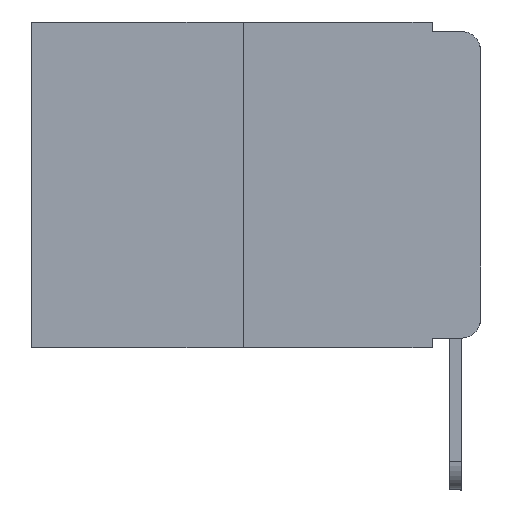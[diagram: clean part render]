
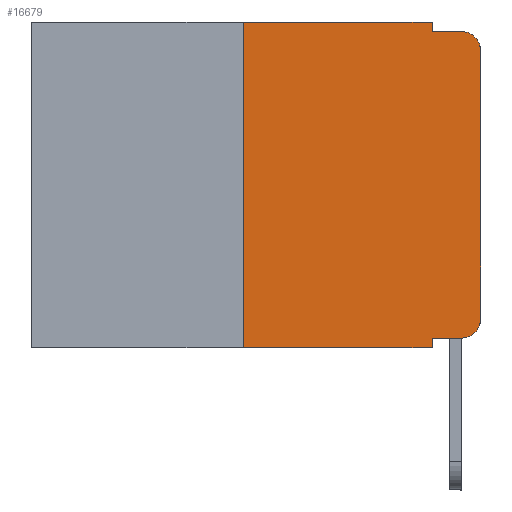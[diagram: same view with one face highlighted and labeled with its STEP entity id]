
A CAD part, left-side view. The second image highlights one B-rep face of the part: STEP entity #16679.
In plain terms, the highlighted planar face has unit normal (-1, 0, 0).
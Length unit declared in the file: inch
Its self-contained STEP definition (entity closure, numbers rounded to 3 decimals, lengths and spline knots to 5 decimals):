
#248 = LINE ( 'NONE', #6428, #6552 ) ;
#523 = EDGE_CURVE ( 'NONE', #12694, #17969, #16596, .T. ) ;
#1305 = VECTOR ( 'NONE', #3465, 39.37008 ) ;
#1343 = DIRECTION ( 'NONE',  ( 0., 0., -1. ) ) ;
#1413 = CARTESIAN_POINT ( 'NONE',  ( 0., 0., -0.03 ) ) ;
#1513 = CARTESIAN_POINT ( 'NONE',  ( 0., 0.473, -0.343 ) ) ;
#1950 = AXIS2_PLACEMENT_3D ( 'NONE', #7630, #7432, #1343 ) ;
#3198 = CARTESIAN_POINT ( 'NONE',  ( 0., 0.02, -0.333 ) ) ;
#3221 = EDGE_CURVE ( 'NONE', #6096, #13166, #12821, .T. ) ;
#3465 = DIRECTION ( 'NONE',  ( 0., 0., -1. ) ) ;
#3627 = ORIENTED_EDGE ( 'NONE', *, *, #523, .F. ) ;
#3660 = CARTESIAN_POINT ( 'NONE',  ( 0., 0.051, 0. ) ) ;
#3879 = CARTESIAN_POINT ( 'NONE',  ( 0., 0.25, -0.343 ) ) ;
#3908 = ORIENTED_EDGE ( 'NONE', *, *, #4370, .F. ) ;
#3960 = CIRCLE ( 'NONE', #19235, 0.02 ) ;
#4212 = CARTESIAN_POINT ( 'NONE',  ( 0., 0.25, 0. ) ) ;
#4370 = EDGE_CURVE ( 'NONE', #14528, #16670, #248, .T. ) ;
#4407 = VECTOR ( 'NONE', #10642, 39.37008 ) ;
#4657 = DIRECTION ( 'NONE',  ( 0., 0., 1. ) ) ;
#4726 = ORIENTED_EDGE ( 'NONE', *, *, #6955, .T. ) ;
#4811 = DIRECTION ( 'NONE',  ( -1., 0., 0. ) ) ;
#5202 = EDGE_CURVE ( 'NONE', #8210, #15841, #7798, .T. ) ;
#5448 = ORIENTED_EDGE ( 'NONE', *, *, #18384, .T. ) ;
#6096 = VERTEX_POINT ( 'NONE', #17494 ) ;
#6428 = CARTESIAN_POINT ( 'NONE',  ( 0., 0.051, 0. ) ) ;
#6497 = CARTESIAN_POINT ( 'NONE',  ( 0., 0.473, 0. ) ) ;
#6552 = VECTOR ( 'NONE', #17311, 39.37008 ) ;
#6747 = EDGE_LOOP ( 'NONE', ( #20002, #5448, #15507, #15849, #15012, #3627, #12566, #3908, #11914, #4726 ) ) ;
#6955 = EDGE_CURVE ( 'NONE', #18101, #8210, #16086, .T. ) ;
#7432 = DIRECTION ( 'NONE',  ( 1., 0., 0. ) ) ;
#7459 = CARTESIAN_POINT ( 'NONE',  ( 0., 0., -0.313 ) ) ;
#7630 = CARTESIAN_POINT ( 'NONE',  ( 0., 0.473, 0. ) ) ;
#7725 = DIRECTION ( 'NONE',  ( 0., -1., 0. ) ) ;
#7746 = CARTESIAN_POINT ( 'NONE',  ( 0., 0.02, -0.313 ) ) ;
#7798 = LINE ( 'NONE', #12476, #10838 ) ;
#8210 = VERTEX_POINT ( 'NONE', #7459 ) ;
#10475 = CARTESIAN_POINT ( 'NONE',  ( 0., 0.051, -0.343 ) ) ;
#10642 = DIRECTION ( 'NONE',  ( 0., -1., 0. ) ) ;
#10838 = VECTOR ( 'NONE', #4657, 39.37008 ) ;
#11497 = CARTESIAN_POINT ( 'NONE',  ( 0., 0.051, -0.01 ) ) ;
#11809 = CARTESIAN_POINT ( 'NONE',  ( 0., 0.25, 0. ) ) ;
#11914 = ORIENTED_EDGE ( 'NONE', *, *, #13280, .T. ) ;
#11916 = DIRECTION ( 'NONE',  ( 0., 0., 1. ) ) ;
#12083 = CARTESIAN_POINT ( 'NONE',  ( 0., 0.02, -0.03 ) ) ;
#12347 = VERTEX_POINT ( 'NONE', #13642 ) ;
#12476 = CARTESIAN_POINT ( 'NONE',  ( 0., 0., 0. ) ) ;
#12566 = ORIENTED_EDGE ( 'NONE', *, *, #13391, .T. ) ;
#12694 = VERTEX_POINT ( 'NONE', #3879 ) ;
#12783 = CARTESIAN_POINT ( 'NONE',  ( 0., 0.02, -0.01 ) ) ;
#12821 = LINE ( 'NONE', #11497, #15847 ) ;
#13166 = VERTEX_POINT ( 'NONE', #12783 ) ;
#13225 = DIRECTION ( 'NONE',  ( 0., -1., 0. ) ) ;
#13280 = EDGE_CURVE ( 'NONE', #14528, #18101, #18278, .T. ) ;
#13391 = EDGE_CURVE ( 'NONE', #12694, #16670, #16845, .T. ) ;
#13642 = CARTESIAN_POINT ( 'NONE',  ( 0., 0.051, 0. ) ) ;
#13929 = FACE_OUTER_BOUND ( 'NONE', #6747, .T. ) ;
#14127 = VECTOR ( 'NONE', #20014, 39.37008 ) ;
#14528 = VERTEX_POINT ( 'NONE', #16440 ) ;
#14786 = AXIS2_PLACEMENT_3D ( 'NONE', #7746, #4811, #17109 ) ;
#15012 = ORIENTED_EDGE ( 'NONE', *, *, #18983, .F. ) ;
#15507 = ORIENTED_EDGE ( 'NONE', *, *, #3221, .F. ) ;
#15657 = LINE ( 'NONE', #3660, #1305 ) ;
#15841 = VERTEX_POINT ( 'NONE', #1413 ) ;
#15847 = VECTOR ( 'NONE', #13225, 39.37008 ) ;
#15849 = ORIENTED_EDGE ( 'NONE', *, *, #16791, .F. ) ;
#16086 = CIRCLE ( 'NONE', #14786, 0.02 ) ;
#16440 = CARTESIAN_POINT ( 'NONE',  ( 0., 0.051, -0.333 ) ) ;
#16460 = CARTESIAN_POINT ( 'NONE',  ( 0., 0.051, -0.333 ) ) ;
#16596 = LINE ( 'NONE', #11809, #17118 ) ;
#16670 = VERTEX_POINT ( 'NONE', #10475 ) ;
#16679 = ADVANCED_FACE ( 'NONE', ( #13929 ), #16788, .F. ) ;
#16788 = PLANE ( 'NONE',  #1950 ) ;
#16791 = EDGE_CURVE ( 'NONE', #12347, #6096, #15657, .T. ) ;
#16845 = LINE ( 'NONE', #1513, #14127 ) ;
#17109 = DIRECTION ( 'NONE',  ( 0., 0., -1. ) ) ;
#17118 = VECTOR ( 'NONE', #11916, 39.37008 ) ;
#17311 = DIRECTION ( 'NONE',  ( 0., 0., -1. ) ) ;
#17494 = CARTESIAN_POINT ( 'NONE',  ( 0., 0.051, -0.01 ) ) ;
#17969 = VERTEX_POINT ( 'NONE', #4212 ) ;
#18101 = VERTEX_POINT ( 'NONE', #3198 ) ;
#18278 = LINE ( 'NONE', #16460, #4407 ) ;
#18296 = DIRECTION ( 'NONE',  ( 0., 0., -1. ) ) ;
#18384 = EDGE_CURVE ( 'NONE', #15841, #13166, #3960, .T. ) ;
#18399 = DIRECTION ( 'NONE',  ( -1., 0., 0. ) ) ;
#18983 = EDGE_CURVE ( 'NONE', #17969, #12347, #20050, .T. ) ;
#19235 = AXIS2_PLACEMENT_3D ( 'NONE', #12083, #18399, #18296 ) ;
#19264 = VECTOR ( 'NONE', #7725, 39.37008 ) ;
#20002 = ORIENTED_EDGE ( 'NONE', *, *, #5202, .T. ) ;
#20014 = DIRECTION ( 'NONE',  ( 0., -1., 0. ) ) ;
#20050 = LINE ( 'NONE', #6497, #19264 ) ;
